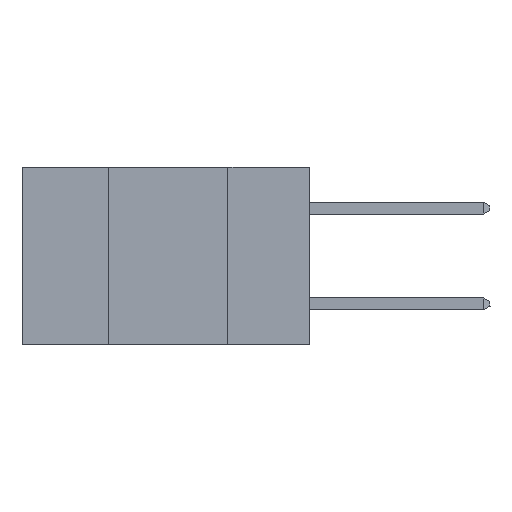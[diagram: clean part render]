
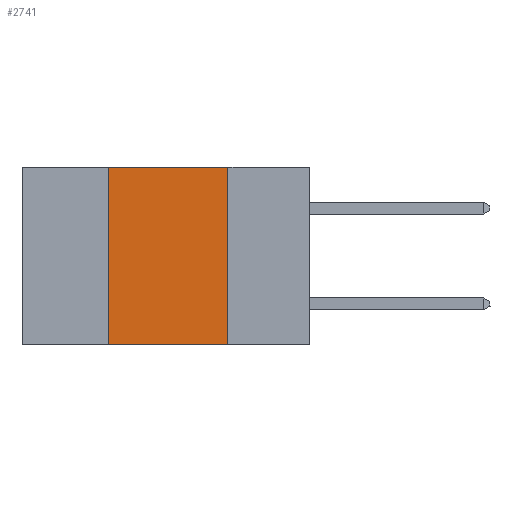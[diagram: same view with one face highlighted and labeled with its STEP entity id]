
A CAD part, left-side view. The second image highlights one B-rep face of the part: STEP entity #2741.
In plain terms, the highlighted planar face has unit normal (-1, 0, 0).
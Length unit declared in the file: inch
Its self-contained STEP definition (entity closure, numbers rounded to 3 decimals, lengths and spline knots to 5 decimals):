
#439 = PLANE ( 'NONE',  #9249 ) ;
#912 = CARTESIAN_POINT ( 'NONE',  ( 0., 0.6, -0.37 ) ) ;
#1088 = VECTOR ( 'NONE', #13423, 39.37008 ) ;
#1153 = DIRECTION ( 'NONE',  ( 0., -1., 0. ) ) ;
#1456 = CARTESIAN_POINT ( 'NONE',  ( 0., 0.17, 0. ) ) ;
#2741 = ADVANCED_FACE ( 'NONE', ( #4024 ), #439, .F. ) ;
#4024 = FACE_OUTER_BOUND ( 'NONE', #6188, .T. ) ;
#4140 = DIRECTION ( 'NONE',  ( 0., 0., -1. ) ) ;
#5552 = VECTOR ( 'NONE', #1153, 39.37008 ) ;
#5685 = LINE ( 'NONE', #19229, #1088 ) ;
#6188 = EDGE_LOOP ( 'NONE', ( #6354, #10369, #17003, #8050 ) ) ;
#6278 = VERTEX_POINT ( 'NONE', #22707 ) ;
#6354 = ORIENTED_EDGE ( 'NONE', *, *, #12921, .F. ) ;
#7289 = CARTESIAN_POINT ( 'NONE',  ( 0., 0.17, 0. ) ) ;
#8050 = ORIENTED_EDGE ( 'NONE', *, *, #25030, .T. ) ;
#8170 = DIRECTION ( 'NONE',  ( 0., 0., 1. ) ) ;
#9239 = VECTOR ( 'NONE', #16830, 39.37008 ) ;
#9249 = AXIS2_PLACEMENT_3D ( 'NONE', #23579, #21757, #4140 ) ;
#9272 = CARTESIAN_POINT ( 'NONE',  ( 0., 0.17, -0.37 ) ) ;
#10369 = ORIENTED_EDGE ( 'NONE', *, *, #17188, .F. ) ;
#11109 = LINE ( 'NONE', #7289, #9239 ) ;
#11902 = EDGE_CURVE ( 'NONE', #6278, #13997, #17576, .T. ) ;
#12921 = EDGE_CURVE ( 'NONE', #18529, #19238, #11109, .T. ) ;
#13423 = DIRECTION ( 'NONE',  ( 0., -1., 0. ) ) ;
#13481 = CARTESIAN_POINT ( 'NONE',  ( 0., 0.42, 0. ) ) ;
#13997 = VERTEX_POINT ( 'NONE', #13481 ) ;
#16830 = DIRECTION ( 'NONE',  ( 0., 0., -1. ) ) ;
#17003 = ORIENTED_EDGE ( 'NONE', *, *, #11902, .F. ) ;
#17188 = EDGE_CURVE ( 'NONE', #13997, #18529, #5685, .T. ) ;
#17576 = LINE ( 'NONE', #21494, #19596 ) ;
#18426 = LINE ( 'NONE', #912, #5552 ) ;
#18529 = VERTEX_POINT ( 'NONE', #1456 ) ;
#19229 = CARTESIAN_POINT ( 'NONE',  ( 0., 0.6, 0. ) ) ;
#19238 = VERTEX_POINT ( 'NONE', #9272 ) ;
#19596 = VECTOR ( 'NONE', #8170, 39.37008 ) ;
#21494 = CARTESIAN_POINT ( 'NONE',  ( 0., 0.42, 0. ) ) ;
#21757 = DIRECTION ( 'NONE',  ( 1., 0., 0. ) ) ;
#22707 = CARTESIAN_POINT ( 'NONE',  ( 0., 0.42, -0.37 ) ) ;
#23579 = CARTESIAN_POINT ( 'NONE',  ( 0., 0.6, 0. ) ) ;
#25030 = EDGE_CURVE ( 'NONE', #6278, #19238, #18426, .T. ) ;
